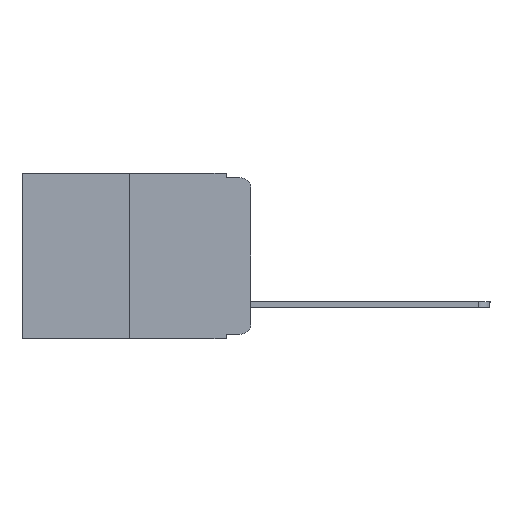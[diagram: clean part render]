
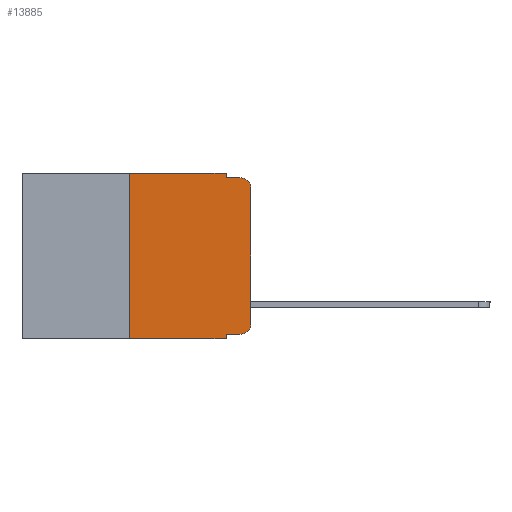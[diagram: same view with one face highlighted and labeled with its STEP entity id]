
A CAD part, left-side view. The second image highlights one B-rep face of the part: STEP entity #13885.
In plain terms, the highlighted planar face has unit normal (-1, 0, 0).
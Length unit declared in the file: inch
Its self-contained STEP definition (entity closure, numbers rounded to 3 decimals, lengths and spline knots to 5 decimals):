
#969 = DIRECTION ( 'NONE',  ( 0., 0., -1. ) ) ;
#1480 = VECTOR ( 'NONE', #6128, 39.37008 ) ;
#1512 = VERTEX_POINT ( 'NONE', #1958 ) ;
#1679 = LINE ( 'NONE', #9645, #5137 ) ;
#1958 = CARTESIAN_POINT ( 'NONE',  ( 0., 0.02, -0.333 ) ) ;
#2432 = EDGE_CURVE ( 'NONE', #5210, #1512, #3623, .T. ) ;
#2589 = ORIENTED_EDGE ( 'NONE', *, *, #20202, .F. ) ;
#2928 = ORIENTED_EDGE ( 'NONE', *, *, #25180, .F. ) ;
#2948 = LINE ( 'NONE', #16728, #12420 ) ;
#3185 = DIRECTION ( 'NONE',  ( -1., 0., 0. ) ) ;
#3265 = EDGE_CURVE ( 'NONE', #5275, #10195, #1679, .T. ) ;
#3338 = CIRCLE ( 'NONE', #17418, 0.02 ) ;
#3493 = VECTOR ( 'NONE', #17876, 39.37008 ) ;
#3623 = LINE ( 'NONE', #11791, #15521 ) ;
#3681 = CARTESIAN_POINT ( 'NONE',  ( 0., 0.051, -0.343 ) ) ;
#4150 = VERTEX_POINT ( 'NONE', #5046 ) ;
#4829 = DIRECTION ( 'NONE',  ( 0., 0., -1. ) ) ;
#5043 = EDGE_CURVE ( 'NONE', #5275, #16717, #6920, .T. ) ;
#5046 = CARTESIAN_POINT ( 'NONE',  ( 0., 0., -0.313 ) ) ;
#5137 = VECTOR ( 'NONE', #11952, 39.37008 ) ;
#5210 = VERTEX_POINT ( 'NONE', #17423 ) ;
#5275 = VERTEX_POINT ( 'NONE', #19367 ) ;
#5325 = ORIENTED_EDGE ( 'NONE', *, *, #5043, .F. ) ;
#6128 = DIRECTION ( 'NONE',  ( 0., 0., -1. ) ) ;
#6845 = DIRECTION ( 'NONE',  ( 0., 0., 1. ) ) ;
#6920 = LINE ( 'NONE', #18599, #18564 ) ;
#6978 = EDGE_CURVE ( 'NONE', #1512, #4150, #3338, .T. ) ;
#7286 = CARTESIAN_POINT ( 'NONE',  ( 0., 0.473, 0. ) ) ;
#7621 = VERTEX_POINT ( 'NONE', #19602 ) ;
#7956 = DIRECTION ( 'NONE',  ( 0., -1., 0. ) ) ;
#8048 = VERTEX_POINT ( 'NONE', #23338 ) ;
#8078 = CARTESIAN_POINT ( 'NONE',  ( 0., 0.051, 0. ) ) ;
#8120 = ORIENTED_EDGE ( 'NONE', *, *, #2432, .T. ) ;
#8272 = CARTESIAN_POINT ( 'NONE',  ( 0., 0.051, -0.01 ) ) ;
#8371 = ORIENTED_EDGE ( 'NONE', *, *, #6978, .T. ) ;
#9246 = FACE_OUTER_BOUND ( 'NONE', #10399, .T. ) ;
#9430 = CARTESIAN_POINT ( 'NONE',  ( 0., 0.02, -0.03 ) ) ;
#9498 = CARTESIAN_POINT ( 'NONE',  ( 0., 0.02, -0.313 ) ) ;
#9645 = CARTESIAN_POINT ( 'NONE',  ( 0., 0.473, -0.343 ) ) ;
#9909 = CARTESIAN_POINT ( 'NONE',  ( 0., 0.473, 0. ) ) ;
#10195 = VERTEX_POINT ( 'NONE', #3681 ) ;
#10235 = LINE ( 'NONE', #11911, #16588 ) ;
#10399 = EDGE_LOOP ( 'NONE', ( #20894, #24499, #10703, #2928, #2589, #5325, #13422, #21088, #8120, #8371 ) ) ;
#10703 = ORIENTED_EDGE ( 'NONE', *, *, #19065, .F. ) ;
#10788 = CARTESIAN_POINT ( 'NONE',  ( 0., 0., -0.03 ) ) ;
#10954 = CARTESIAN_POINT ( 'NONE',  ( 0., 0.25, 0. ) ) ;
#11184 = DIRECTION ( 'NONE',  ( 0., 0., -1. ) ) ;
#11551 = VERTEX_POINT ( 'NONE', #8078 ) ;
#11791 = CARTESIAN_POINT ( 'NONE',  ( 0., 0.051, -0.333 ) ) ;
#11911 = CARTESIAN_POINT ( 'NONE',  ( 0., 0.051, 0. ) ) ;
#11952 = DIRECTION ( 'NONE',  ( 0., -1., 0. ) ) ;
#12420 = VECTOR ( 'NONE', #6845, 39.37008 ) ;
#13422 = ORIENTED_EDGE ( 'NONE', *, *, #3265, .T. ) ;
#13861 = LINE ( 'NONE', #8272, #3493 ) ;
#13885 = ADVANCED_FACE ( 'NONE', ( #9246 ), #25083, .F. ) ;
#14087 = AXIS2_PLACEMENT_3D ( 'NONE', #7286, #15196, #4829 ) ;
#14428 = LINE ( 'NONE', #22360, #1480 ) ;
#14581 = DIRECTION ( 'NONE',  ( 0., 0., 1. ) ) ;
#14941 = DIRECTION ( 'NONE',  ( -1., 0., 0. ) ) ;
#15196 = DIRECTION ( 'NONE',  ( 1., 0., 0. ) ) ;
#15521 = VECTOR ( 'NONE', #25564, 39.37008 ) ;
#15872 = LINE ( 'NONE', #9909, #25123 ) ;
#16333 = DIRECTION ( 'NONE',  ( 0., 0., -1. ) ) ;
#16588 = VECTOR ( 'NONE', #16333, 39.37008 ) ;
#16717 = VERTEX_POINT ( 'NONE', #10954 ) ;
#16728 = CARTESIAN_POINT ( 'NONE',  ( 0., 0., 0. ) ) ;
#16823 = AXIS2_PLACEMENT_3D ( 'NONE', #9430, #3185, #969 ) ;
#17418 = AXIS2_PLACEMENT_3D ( 'NONE', #9498, #14941, #11184 ) ;
#17423 = CARTESIAN_POINT ( 'NONE',  ( 0., 0.051, -0.333 ) ) ;
#17637 = CIRCLE ( 'NONE', #16823, 0.02 ) ;
#17876 = DIRECTION ( 'NONE',  ( 0., -1., 0. ) ) ;
#18564 = VECTOR ( 'NONE', #14581, 39.37008 ) ;
#18599 = CARTESIAN_POINT ( 'NONE',  ( 0., 0.25, 0. ) ) ;
#19065 = EDGE_CURVE ( 'NONE', #7621, #8048, #13861, .T. ) ;
#19367 = CARTESIAN_POINT ( 'NONE',  ( 0., 0.25, -0.343 ) ) ;
#19602 = CARTESIAN_POINT ( 'NONE',  ( 0., 0.051, -0.01 ) ) ;
#19676 = EDGE_CURVE ( 'NONE', #24880, #8048, #17637, .T. ) ;
#20202 = EDGE_CURVE ( 'NONE', #16717, #11551, #15872, .T. ) ;
#20415 = EDGE_CURVE ( 'NONE', #5210, #10195, #14428, .T. ) ;
#20894 = ORIENTED_EDGE ( 'NONE', *, *, #25288, .T. ) ;
#21088 = ORIENTED_EDGE ( 'NONE', *, *, #20415, .F. ) ;
#22360 = CARTESIAN_POINT ( 'NONE',  ( 0., 0.051, 0. ) ) ;
#23338 = CARTESIAN_POINT ( 'NONE',  ( 0., 0.02, -0.01 ) ) ;
#24499 = ORIENTED_EDGE ( 'NONE', *, *, #19676, .T. ) ;
#24880 = VERTEX_POINT ( 'NONE', #10788 ) ;
#25083 = PLANE ( 'NONE',  #14087 ) ;
#25123 = VECTOR ( 'NONE', #7956, 39.37008 ) ;
#25180 = EDGE_CURVE ( 'NONE', #11551, #7621, #10235, .T. ) ;
#25288 = EDGE_CURVE ( 'NONE', #4150, #24880, #2948, .T. ) ;
#25564 = DIRECTION ( 'NONE',  ( 0., -1., 0. ) ) ;
